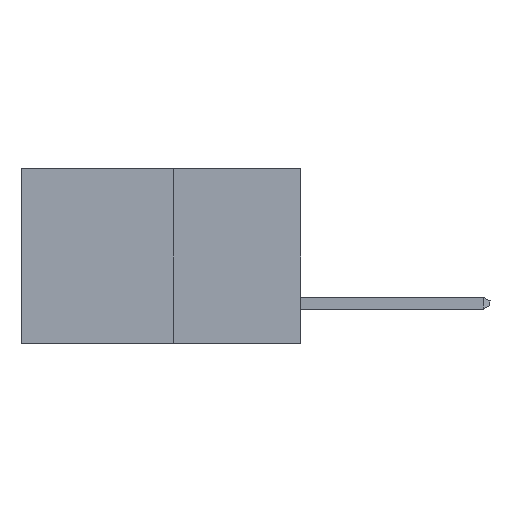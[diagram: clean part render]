
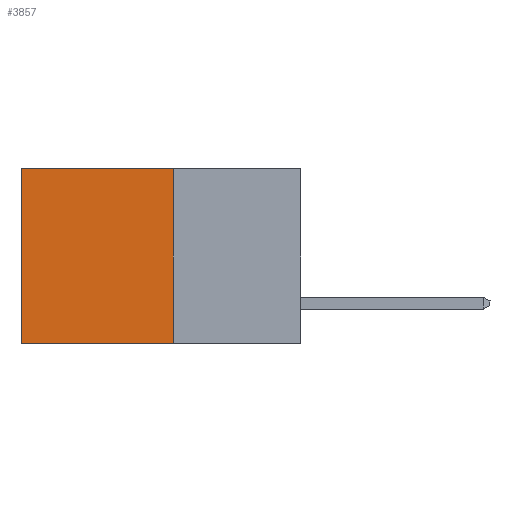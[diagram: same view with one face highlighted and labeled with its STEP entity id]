
A CAD part, left-side view. The second image highlights one B-rep face of the part: STEP entity #3857.
In plain terms, the highlighted planar face has unit normal (-1, 0, 0).
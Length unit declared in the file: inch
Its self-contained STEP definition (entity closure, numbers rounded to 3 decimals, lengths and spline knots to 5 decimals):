
#287 = ORIENTED_EDGE ( 'NONE', *, *, #3975, .T. ) ;
#326 = ORIENTED_EDGE ( 'NONE', *, *, #10508, .F. ) ;
#364 = ORIENTED_EDGE ( 'NONE', *, *, #7714, .F. ) ;
#448 = ORIENTED_EDGE ( 'NONE', *, *, #7615, .T. ) ;
#1332 = LINE ( 'NONE', #10972, #3822 ) ;
#1597 = EDGE_LOOP ( 'NONE', ( #287, #326, #364, #448 ) ) ;
#1947 = DIRECTION ( 'NONE',  ( 0., 1., 0. ) ) ;
#3059 = VECTOR ( 'NONE', #11351, 39.37008 ) ;
#3822 = VECTOR ( 'NONE', #4934, 39.37008 ) ;
#3857 = ADVANCED_FACE ( 'NONE', ( #13188 ), #7303, .F. ) ;
#3975 = EDGE_CURVE ( 'NONE', #6924, #6992, #1332, .T. ) ;
#4207 = CARTESIAN_POINT ( 'NONE',  ( 0.277, 0.27, -0.37 ) ) ;
#4382 = CARTESIAN_POINT ( 'NONE',  ( 0.277, 0.59, -0.37 ) ) ;
#4530 = DIRECTION ( 'NONE',  ( 1., 0., 0. ) ) ;
#4934 = DIRECTION ( 'NONE',  ( 0., 0., -1. ) ) ;
#4980 = LINE ( 'NONE', #8129, #12473 ) ;
#5702 = DIRECTION ( 'NONE',  ( 0., 1., 0. ) ) ;
#6113 = AXIS2_PLACEMENT_3D ( 'NONE', #4207, #4530, #13308 ) ;
#6345 = CARTESIAN_POINT ( 'NONE',  ( 0.277, 0.59, 0. ) ) ;
#6476 = VERTEX_POINT ( 'NONE', #9106 ) ;
#6924 = VERTEX_POINT ( 'NONE', #6345 ) ;
#6992 = VERTEX_POINT ( 'NONE', #4382 ) ;
#7303 = PLANE ( 'NONE',  #6113 ) ;
#7546 = LINE ( 'NONE', #11824, #10604 ) ;
#7615 = EDGE_CURVE ( 'NONE', #10045, #6924, #4980, .T. ) ;
#7714 = EDGE_CURVE ( 'NONE', #10045, #6476, #8490, .T. ) ;
#8129 = CARTESIAN_POINT ( 'NONE',  ( 0.277, 0.27, 0. ) ) ;
#8490 = LINE ( 'NONE', #10318, #3059 ) ;
#9106 = CARTESIAN_POINT ( 'NONE',  ( 0.277, 0.27, -0.37 ) ) ;
#10045 = VERTEX_POINT ( 'NONE', #12470 ) ;
#10318 = CARTESIAN_POINT ( 'NONE',  ( 0.277, 0.27, -0.37 ) ) ;
#10508 = EDGE_CURVE ( 'NONE', #6476, #6992, #7546, .T. ) ;
#10604 = VECTOR ( 'NONE', #5702, 39.37008 ) ;
#10972 = CARTESIAN_POINT ( 'NONE',  ( 0.277, 0.59, -0.37 ) ) ;
#11351 = DIRECTION ( 'NONE',  ( 0., 0., -1. ) ) ;
#11824 = CARTESIAN_POINT ( 'NONE',  ( 0.277, 0.27, -0.37 ) ) ;
#12470 = CARTESIAN_POINT ( 'NONE',  ( 0.277, 0.27, 0. ) ) ;
#12473 = VECTOR ( 'NONE', #1947, 39.37008 ) ;
#13188 = FACE_OUTER_BOUND ( 'NONE', #1597, .T. ) ;
#13308 = DIRECTION ( 'NONE',  ( 0., 0., -1. ) ) ;
